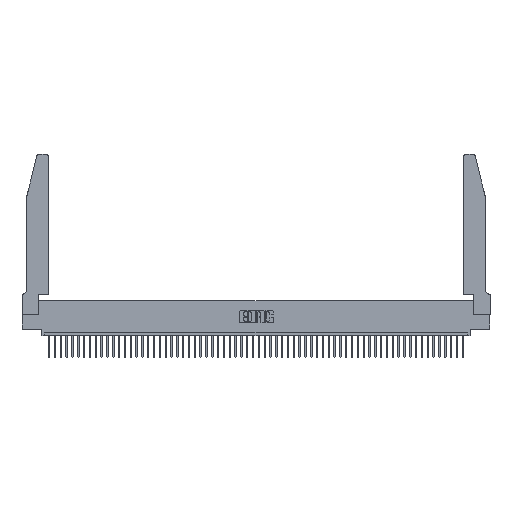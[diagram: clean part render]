
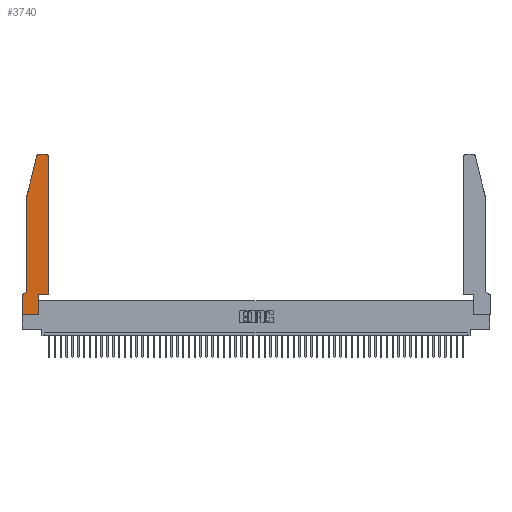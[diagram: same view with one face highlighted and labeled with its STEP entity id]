
A CAD part, top view. The second image highlights one B-rep face of the part: STEP entity #3740.
In plain terms, the highlighted planar face has unit normal (0, 0, 1).
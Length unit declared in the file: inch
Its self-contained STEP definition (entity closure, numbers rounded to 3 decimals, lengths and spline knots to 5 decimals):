
#67 = EDGE_CURVE ( 'NONE', #31194, #45896, #53626, .T. ) ;
#747 = VERTEX_POINT ( 'NONE', #29738 ) ;
#805 = DIRECTION ( 'NONE',  ( -1., 0., 0. ) ) ;
#1048 = CARTESIAN_POINT ( 'NONE',  ( 0.0055, 0.42, 0.37 ) ) ;
#1229 = VECTOR ( 'NONE', #31736, 39.37008 ) ;
#2936 = VECTOR ( 'NONE', #46228, 39.37008 ) ;
#3572 = VERTEX_POINT ( 'NONE', #33502 ) ;
#3740 = ADVANCED_FACE ( 'NONE', ( #23157 ), #19880, .T. ) ;
#3749 = VERTEX_POINT ( 'NONE', #29975 ) ;
#4262 = CARTESIAN_POINT ( 'NONE',  ( 0., 0.35, 0.37 ) ) ;
#4535 = EDGE_CURVE ( 'NONE', #45896, #46130, #19782, .T. ) ;
#5076 = AXIS2_PLACEMENT_3D ( 'NONE', #35656, #39933, #18796 ) ;
#6988 = ORIENTED_EDGE ( 'NONE', *, *, #23824, .T. ) ;
#7461 = DIRECTION ( 'NONE',  ( 1., 0., 0. ) ) ;
#7581 = CARTESIAN_POINT ( 'NONE',  ( 0.0055, 0.35, 0.37 ) ) ;
#7646 = DIRECTION ( 'NONE',  ( 0., 0., 1. ) ) ;
#7924 = EDGE_CURVE ( 'NONE', #13771, #28983, #25144, .T. ) ;
#7929 = VECTOR ( 'NONE', #8609, 39.37008 ) ;
#8609 = DIRECTION ( 'NONE',  ( -0.239, -0.971, 0. ) ) ;
#8662 = AXIS2_PLACEMENT_3D ( 'NONE', #45163, #7646, #7461 ) ;
#9025 = VECTOR ( 'NONE', #43962, 39.37008 ) ;
#9434 = EDGE_CURVE ( 'NONE', #28983, #32909, #9747, .T. ) ;
#9693 = CARTESIAN_POINT ( 'NONE',  ( 0.2865, 0.35, 0.37 ) ) ;
#9747 = LINE ( 'NONE', #11675, #43623 ) ;
#10262 = CARTESIAN_POINT ( 'NONE',  ( 0.0755, 2., 0.37 ) ) ;
#10968 = ORIENTED_EDGE ( 'NONE', *, *, #67, .T. ) ;
#11307 = CIRCLE ( 'NONE', #5076, 0.03 ) ;
#11598 = ORIENTED_EDGE ( 'NONE', *, *, #41965, .T. ) ;
#11675 = CARTESIAN_POINT ( 'NONE',  ( 0.0755, 2., 0.37 ) ) ;
#12178 = EDGE_CURVE ( 'NONE', #747, #13771, #40034, .T. ) ;
#12971 = VERTEX_POINT ( 'NONE', #51166 ) ;
#13363 = CARTESIAN_POINT ( 'NONE',  ( 0.0755, 2., 0.37 ) ) ;
#13423 = VECTOR ( 'NONE', #805, 39.37008 ) ;
#13771 = VERTEX_POINT ( 'NONE', #48492 ) ;
#14189 = LINE ( 'NONE', #16118, #2936 ) ;
#14821 = CARTESIAN_POINT ( 'NONE',  ( 0., 0., 0.37 ) ) ;
#15495 = DIRECTION ( 'NONE',  ( 1., 0., 0. ) ) ;
#16118 = CARTESIAN_POINT ( 'NONE',  ( 0.4505, 0.35, 0.37 ) ) ;
#16899 = CARTESIAN_POINT ( 'NONE',  ( 0.0755, 0.35, 0.37 ) ) ;
#17600 = DIRECTION ( 'NONE',  ( 0., 0., 1. ) ) ;
#18796 = DIRECTION ( 'NONE',  ( 1., 0., 0. ) ) ;
#19782 = LINE ( 'NONE', #9693, #26336 ) ;
#19880 = PLANE ( 'NONE',  #32566 ) ;
#20809 = LINE ( 'NONE', #54637, #23399 ) ;
#21376 = ORIENTED_EDGE ( 'NONE', *, *, #4535, .T. ) ;
#23157 = FACE_OUTER_BOUND ( 'NONE', #30510, .T. ) ;
#23399 = VECTOR ( 'NONE', #47839, 39.37008 ) ;
#23824 = EDGE_CURVE ( 'NONE', #12971, #31194, #20809, .T. ) ;
#23925 = CARTESIAN_POINT ( 'NONE',  ( 0.0755, 0.42, 0.37 ) ) ;
#24977 = VECTOR ( 'NONE', #43797, 39.37008 ) ;
#25144 = LINE ( 'NONE', #13363, #7929 ) ;
#25156 = ORIENTED_EDGE ( 'NONE', *, *, #34785, .T. ) ;
#25738 = ORIENTED_EDGE ( 'NONE', *, *, #9434, .T. ) ;
#26336 = VECTOR ( 'NONE', #32500, 39.37008 ) ;
#28983 = VERTEX_POINT ( 'NONE', #10262 ) ;
#29403 = CARTESIAN_POINT ( 'NONE',  ( 0.2865, 0., 0.37 ) ) ;
#29738 = CARTESIAN_POINT ( 'NONE',  ( 0.284, 2.75, 0.37 ) ) ;
#29975 = CARTESIAN_POINT ( 'NONE',  ( 0.4505, 2.72, 0.37 ) ) ;
#30323 = CARTESIAN_POINT ( 'NONE',  ( 0.2865, 0.35, 0.37 ) ) ;
#30510 = EDGE_LOOP ( 'NONE', ( #54844, #47362, #39123, #25738, #32585, #11598, #6988, #10968, #21376, #35046, #25156, #34665 ) ) ;
#30925 = CARTESIAN_POINT ( 'NONE',  ( 0.4505, 0.35, 0.37 ) ) ;
#31194 = VERTEX_POINT ( 'NONE', #14821 ) ;
#31723 = EDGE_CURVE ( 'NONE', #3572, #747, #48539, .T. ) ;
#31736 = DIRECTION ( 'NONE',  ( -1., 0., 0. ) ) ;
#31749 = EDGE_CURVE ( 'NONE', #3749, #3572, #11307, .T. ) ;
#32500 = DIRECTION ( 'NONE',  ( 0., 1., 0. ) ) ;
#32566 = AXIS2_PLACEMENT_3D ( 'NONE', #4262, #17600, #15495 ) ;
#32585 = ORIENTED_EDGE ( 'NONE', *, *, #50760, .T. ) ;
#32909 = VERTEX_POINT ( 'NONE', #23925 ) ;
#33502 = CARTESIAN_POINT ( 'NONE',  ( 0.4205, 2.75, 0.37 ) ) ;
#33708 = CIRCLE ( 'NONE', #46985, 0.07 ) ;
#34665 = ORIENTED_EDGE ( 'NONE', *, *, #31749, .T. ) ;
#34785 = EDGE_CURVE ( 'NONE', #45568, #3749, #36303, .T. ) ;
#35046 = ORIENTED_EDGE ( 'NONE', *, *, #41101, .T. ) ;
#35656 = CARTESIAN_POINT ( 'NONE',  ( 0.4205, 2.72, 0.37 ) ) ;
#36053 = LINE ( 'NONE', #16899, #13423 ) ;
#36303 = LINE ( 'NONE', #30925, #24977 ) ;
#39123 = ORIENTED_EDGE ( 'NONE', *, *, #7924, .T. ) ;
#39933 = DIRECTION ( 'NONE',  ( 0., 0., 1. ) ) ;
#40034 = CIRCLE ( 'NONE', #8662, 0.03 ) ;
#41101 = EDGE_CURVE ( 'NONE', #46130, #45568, #14189, .T. ) ;
#41890 = DIRECTION ( 'NONE',  ( 0., -1., 0. ) ) ;
#41965 = EDGE_CURVE ( 'NONE', #53962, #12971, #36053, .T. ) ;
#43077 = DIRECTION ( 'NONE',  ( 0., 0., -1. ) ) ;
#43623 = VECTOR ( 'NONE', #41890, 39.37008 ) ;
#43797 = DIRECTION ( 'NONE',  ( 0., 1., 0. ) ) ;
#43962 = DIRECTION ( 'NONE',  ( 1., 0., 0. ) ) ;
#45163 = CARTESIAN_POINT ( 'NONE',  ( 0.284, 2.72, 0.37 ) ) ;
#45568 = VERTEX_POINT ( 'NONE', #52274 ) ;
#45896 = VERTEX_POINT ( 'NONE', #29403 ) ;
#46130 = VERTEX_POINT ( 'NONE', #30323 ) ;
#46228 = DIRECTION ( 'NONE',  ( 1., 0., 0. ) ) ;
#46985 = AXIS2_PLACEMENT_3D ( 'NONE', #1048, #43077, #47411 ) ;
#47362 = ORIENTED_EDGE ( 'NONE', *, *, #12178, .T. ) ;
#47411 = DIRECTION ( 'NONE',  ( -1., 0., 0. ) ) ;
#47839 = DIRECTION ( 'NONE',  ( 0., -1., 0. ) ) ;
#48090 = CARTESIAN_POINT ( 'NONE',  ( 0., 0., 0.37 ) ) ;
#48492 = CARTESIAN_POINT ( 'NONE',  ( 0.25487, 2.72718, 0.37 ) ) ;
#48539 = LINE ( 'NONE', #52232, #1229 ) ;
#50760 = EDGE_CURVE ( 'NONE', #32909, #53962, #33708, .T. ) ;
#51166 = CARTESIAN_POINT ( 'NONE',  ( 0., 0.35, 0.37 ) ) ;
#52232 = CARTESIAN_POINT ( 'NONE',  ( 0.2605, 2.75, 0.37 ) ) ;
#52274 = CARTESIAN_POINT ( 'NONE',  ( 0.4505, 0.35, 0.37 ) ) ;
#53626 = LINE ( 'NONE', #48090, #9025 ) ;
#53962 = VERTEX_POINT ( 'NONE', #7581 ) ;
#54637 = CARTESIAN_POINT ( 'NONE',  ( 0., 0., 0.37 ) ) ;
#54844 = ORIENTED_EDGE ( 'NONE', *, *, #31723, .T. ) ;
